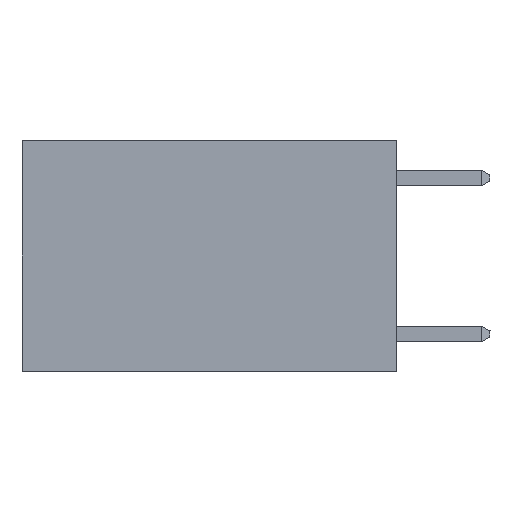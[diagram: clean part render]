
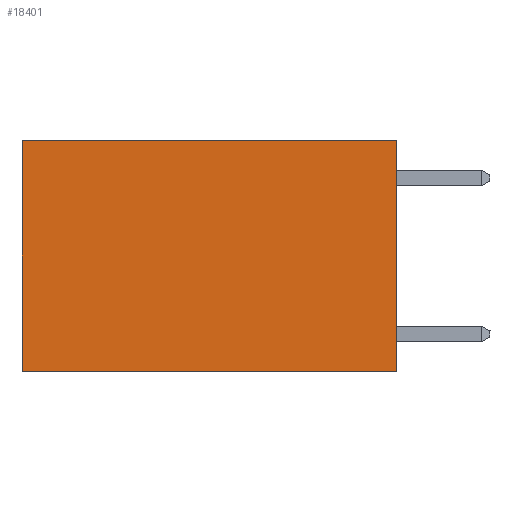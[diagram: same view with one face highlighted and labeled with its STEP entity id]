
A CAD part, left-side view. The second image highlights one B-rep face of the part: STEP entity #18401.
In plain terms, the highlighted planar face has unit normal (-1, 0, 0).
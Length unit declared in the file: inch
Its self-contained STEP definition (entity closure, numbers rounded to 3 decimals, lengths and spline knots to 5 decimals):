
#1010 = CARTESIAN_POINT ( 'NONE',  ( 0.2625, 0., 0. ) ) ;
#1988 = CARTESIAN_POINT ( 'NONE',  ( 0.2625, 0., -0.37 ) ) ;
#2566 = VECTOR ( 'NONE', #19122, 39.37008 ) ;
#2573 = LINE ( 'NONE', #23357, #2566 ) ;
#3023 = ORIENTED_EDGE ( 'NONE', *, *, #15329, .T. ) ;
#3266 = DIRECTION ( 'NONE',  ( 1., 0., 0. ) ) ;
#4756 = AXIS2_PLACEMENT_3D ( 'NONE', #1010, #3266, #18446 ) ;
#5246 = ORIENTED_EDGE ( 'NONE', *, *, #8489, .F. ) ;
#6316 = EDGE_CURVE ( 'NONE', #15268, #18984, #7348, .T. ) ;
#6818 = VERTEX_POINT ( 'NONE', #11024 ) ;
#7176 = VECTOR ( 'NONE', #8865, 39.37008 ) ;
#7348 = LINE ( 'NONE', #9039, #7377 ) ;
#7377 = VECTOR ( 'NONE', #11147, 39.37008 ) ;
#7412 = LINE ( 'NONE', #25746, #7176 ) ;
#8489 = EDGE_CURVE ( 'NONE', #22648, #18984, #7412, .T. ) ;
#8865 = DIRECTION ( 'NONE',  ( 0., 1., 0. ) ) ;
#9039 = CARTESIAN_POINT ( 'NONE',  ( 0.2625, 0.6, 0. ) ) ;
#9371 = CARTESIAN_POINT ( 'NONE',  ( 0.2625, 0., 0. ) ) ;
#9773 = CARTESIAN_POINT ( 'NONE',  ( 0.2625, 0.6, -0.37 ) ) ;
#11024 = CARTESIAN_POINT ( 'NONE',  ( 0.2625, 0., 0. ) ) ;
#11147 = DIRECTION ( 'NONE',  ( 0., 0., -1. ) ) ;
#13134 = ORIENTED_EDGE ( 'NONE', *, *, #6316, .T. ) ;
#15268 = VERTEX_POINT ( 'NONE', #20979 ) ;
#15329 = EDGE_CURVE ( 'NONE', #6818, #15268, #2573, .T. ) ;
#16249 = VECTOR ( 'NONE', #22097, 39.37008 ) ;
#18401 = ADVANCED_FACE ( 'NONE', ( #26502 ), #26691, .F. ) ;
#18446 = DIRECTION ( 'NONE',  ( 0., 0., -1. ) ) ;
#18918 = EDGE_LOOP ( 'NONE', ( #13134, #5246, #25534, #3023 ) ) ;
#18984 = VERTEX_POINT ( 'NONE', #9773 ) ;
#19122 = DIRECTION ( 'NONE',  ( 0., 1., 0. ) ) ;
#20979 = CARTESIAN_POINT ( 'NONE',  ( 0.2625, 0.6, 0. ) ) ;
#21577 = EDGE_CURVE ( 'NONE', #6818, #22648, #26640, .T. ) ;
#22097 = DIRECTION ( 'NONE',  ( 0., 0., -1. ) ) ;
#22648 = VERTEX_POINT ( 'NONE', #1988 ) ;
#23357 = CARTESIAN_POINT ( 'NONE',  ( 0.2625, 0., 0. ) ) ;
#25534 = ORIENTED_EDGE ( 'NONE', *, *, #21577, .F. ) ;
#25746 = CARTESIAN_POINT ( 'NONE',  ( 0.2625, 0., -0.37 ) ) ;
#26502 = FACE_OUTER_BOUND ( 'NONE', #18918, .T. ) ;
#26640 = LINE ( 'NONE', #9371, #16249 ) ;
#26691 = PLANE ( 'NONE',  #4756 ) ;
